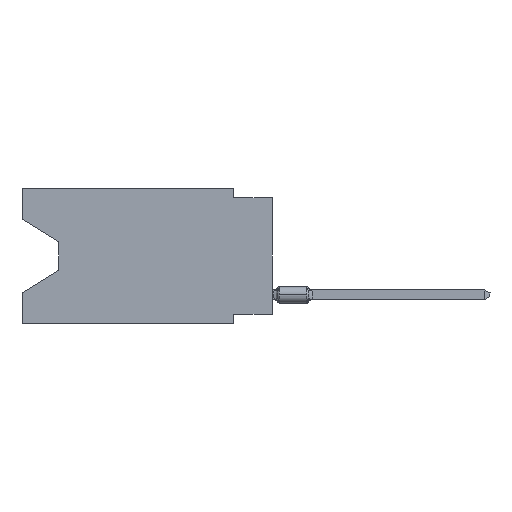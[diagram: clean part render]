
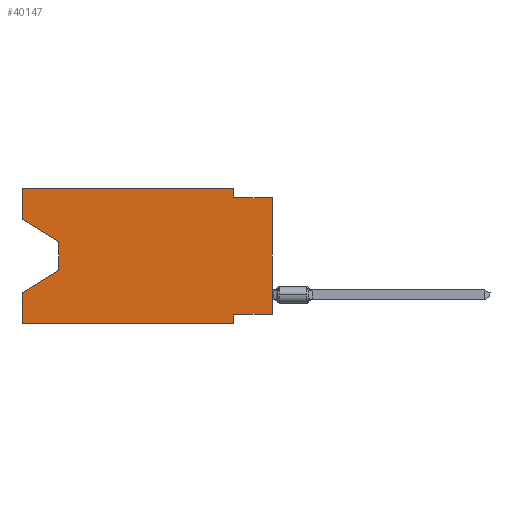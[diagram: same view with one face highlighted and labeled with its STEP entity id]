
A CAD part, left-side view. The second image highlights one B-rep face of the part: STEP entity #40147.
In plain terms, the highlighted planar face has unit normal (-1, 0, 0).
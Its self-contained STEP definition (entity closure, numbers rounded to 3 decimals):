
#376 = DIRECTION ( 'NONE',  ( 0., 0.855, -0.519 ) ) ;
#2074 = EDGE_CURVE ( 'NONE', #8241, #29159, #5861, .T. ) ;
#2849 = CARTESIAN_POINT ( 'NONE',  ( 0., 16.383, -6.852 ) ) ;
#2968 = CARTESIAN_POINT ( 'NONE',  ( 0., 16.383, 0. ) ) ;
#3019 = EDGE_CURVE ( 'NONE', #36247, #46033, #17302, .T. ) ;
#3469 = ORIENTED_EDGE ( 'NONE', *, *, #37032, .T. ) ;
#3727 = CARTESIAN_POINT ( 'NONE',  ( 0., 13.97, -5.385 ) ) ;
#4745 = VERTEX_POINT ( 'NONE', #33444 ) ;
#4913 = CARTESIAN_POINT ( 'NONE',  ( 0., 2.54, -0.635 ) ) ;
#5861 = LINE ( 'NONE', #44570, #18632 ) ;
#6766 = VECTOR ( 'NONE', #48498, 1000. ) ;
#6932 = EDGE_CURVE ( 'NONE', #23714, #14240, #28679, .T. ) ;
#8034 = CARTESIAN_POINT ( 'NONE',  ( 0., 16.383, -8.89 ) ) ;
#8043 = DIRECTION ( 'NONE',  ( 0., 0., -1. ) ) ;
#8229 = VERTEX_POINT ( 'NONE', #39587 ) ;
#8241 = VERTEX_POINT ( 'NONE', #35573 ) ;
#8360 = ORIENTED_EDGE ( 'NONE', *, *, #20843, .T. ) ;
#8700 = AXIS2_PLACEMENT_3D ( 'NONE', #2968, #31608, #11507 ) ;
#9347 = CARTESIAN_POINT ( 'NONE',  ( 0., 16.383, 0. ) ) ;
#9690 = ORIENTED_EDGE ( 'NONE', *, *, #22733, .F. ) ;
#9769 = DIRECTION ( 'NONE',  ( 0., 0., -1. ) ) ;
#10174 = CARTESIAN_POINT ( 'NONE',  ( 0., 0., 0. ) ) ;
#10528 = FACE_OUTER_BOUND ( 'NONE', #45852, .T. ) ;
#10813 = VECTOR ( 'NONE', #36239, 1000. ) ;
#11239 = ORIENTED_EDGE ( 'NONE', *, *, #6932, .F. ) ;
#11507 = DIRECTION ( 'NONE',  ( 0., 0., -1. ) ) ;
#11816 = LINE ( 'NONE', #42480, #31564 ) ;
#14240 = VERTEX_POINT ( 'NONE', #2849 ) ;
#14755 = EDGE_CURVE ( 'NONE', #29159, #14240, #19476, .T. ) ;
#15243 = VECTOR ( 'NONE', #36760, 1000. ) ;
#15750 = ORIENTED_EDGE ( 'NONE', *, *, #35607, .T. ) ;
#16802 = CARTESIAN_POINT ( 'NONE',  ( 0., 2.54, -8.89 ) ) ;
#17302 = LINE ( 'NONE', #44196, #18596 ) ;
#17561 = DIRECTION ( 'NONE',  ( 0., -1., 0. ) ) ;
#18596 = VECTOR ( 'NONE', #17561, 1000. ) ;
#18632 = VECTOR ( 'NONE', #21186, 1000. ) ;
#19333 = ORIENTED_EDGE ( 'NONE', *, *, #14755, .T. ) ;
#19476 = LINE ( 'NONE', #34807, #44686 ) ;
#20001 = CARTESIAN_POINT ( 'NONE',  ( 0., 16.383, 0. ) ) ;
#20843 = EDGE_CURVE ( 'NONE', #23714, #33346, #42471, .T. ) ;
#20923 = ORIENTED_EDGE ( 'NONE', *, *, #45605, .F. ) ;
#21057 = CARTESIAN_POINT ( 'NONE',  ( 0., 2.54, -8.89 ) ) ;
#21186 = DIRECTION ( 'NONE',  ( 0., 0., -1. ) ) ;
#21317 = DIRECTION ( 'NONE',  ( 0., -1., 0. ) ) ;
#22002 = EDGE_CURVE ( 'NONE', #8229, #36247, #11816, .T. ) ;
#22342 = VECTOR ( 'NONE', #21317, 1000. ) ;
#22733 = EDGE_CURVE ( 'NONE', #4745, #39158, #35975, .T. ) ;
#23513 = ORIENTED_EDGE ( 'NONE', *, *, #25412, .F. ) ;
#23714 = VERTEX_POINT ( 'NONE', #39751 ) ;
#25077 = LINE ( 'NONE', #40437, #22342 ) ;
#25412 = EDGE_CURVE ( 'NONE', #41017, #36835, #32747, .T. ) ;
#25479 = DIRECTION ( 'NONE',  ( 0., 0., 1. ) ) ;
#25672 = CARTESIAN_POINT ( 'NONE',  ( 0., 2.54, -8.255 ) ) ;
#25822 = PLANE ( 'NONE',  #8700 ) ;
#27395 = CARTESIAN_POINT ( 'NONE',  ( 0., 16.383, -2.038 ) ) ;
#27652 = LINE ( 'NONE', #27395, #29356 ) ;
#28679 = LINE ( 'NONE', #9347, #10813 ) ;
#29159 = VERTEX_POINT ( 'NONE', #3727 ) ;
#29356 = VECTOR ( 'NONE', #31698, 1000. ) ;
#29930 = VECTOR ( 'NONE', #47234, 1000. ) ;
#30424 = CARTESIAN_POINT ( 'NONE',  ( 0., 0., -8.255 ) ) ;
#31564 = VECTOR ( 'NONE', #8043, 1000. ) ;
#31608 = DIRECTION ( 'NONE',  ( 1., 0., 0. ) ) ;
#31698 = DIRECTION ( 'NONE',  ( 0., -0.855, -0.519 ) ) ;
#32747 = LINE ( 'NONE', #37244, #15243 ) ;
#33183 = CARTESIAN_POINT ( 'NONE',  ( 0., 16.383, 0. ) ) ;
#33346 = VERTEX_POINT ( 'NONE', #16802 ) ;
#33386 = VECTOR ( 'NONE', #25479, 1000. ) ;
#33444 = CARTESIAN_POINT ( 'NONE',  ( 0., 16.383, -2.038 ) ) ;
#34807 = CARTESIAN_POINT ( 'NONE',  ( 0., 13.97, -5.385 ) ) ;
#35027 = ORIENTED_EDGE ( 'NONE', *, *, #2074, .T. ) ;
#35573 = CARTESIAN_POINT ( 'NONE',  ( 0., 13.97, -3.505 ) ) ;
#35607 = EDGE_CURVE ( 'NONE', #41017, #46033, #44588, .T. ) ;
#35637 = ORIENTED_EDGE ( 'NONE', *, *, #45302, .F. ) ;
#35807 = CARTESIAN_POINT ( 'NONE',  ( 0., 0., -0.635 ) ) ;
#35975 = LINE ( 'NONE', #33183, #6766 ) ;
#36239 = DIRECTION ( 'NONE',  ( 0., 0., 1. ) ) ;
#36247 = VERTEX_POINT ( 'NONE', #4913 ) ;
#36760 = DIRECTION ( 'NONE',  ( 0., 1., 0. ) ) ;
#36835 = VERTEX_POINT ( 'NONE', #25672 ) ;
#37032 = EDGE_CURVE ( 'NONE', #4745, #8241, #27652, .T. ) ;
#37244 = CARTESIAN_POINT ( 'NONE',  ( 0., 0., -8.255 ) ) ;
#39158 = VERTEX_POINT ( 'NONE', #20001 ) ;
#39587 = CARTESIAN_POINT ( 'NONE',  ( 0., 2.54, 0. ) ) ;
#39751 = CARTESIAN_POINT ( 'NONE',  ( 0., 16.383, -8.89 ) ) ;
#40147 = ADVANCED_FACE ( 'NONE', ( #10528 ), #25822, .F. ) ;
#40437 = CARTESIAN_POINT ( 'NONE',  ( 0., 16.383, 0. ) ) ;
#41017 = VERTEX_POINT ( 'NONE', #30424 ) ;
#41159 = LINE ( 'NONE', #21057, #45660 ) ;
#42471 = LINE ( 'NONE', #8034, #29930 ) ;
#42480 = CARTESIAN_POINT ( 'NONE',  ( 0., 2.54, 0. ) ) ;
#44196 = CARTESIAN_POINT ( 'NONE',  ( 0., 0., -0.635 ) ) ;
#44409 = ORIENTED_EDGE ( 'NONE', *, *, #22002, .F. ) ;
#44570 = CARTESIAN_POINT ( 'NONE',  ( 0., 13.97, -3.505 ) ) ;
#44588 = LINE ( 'NONE', #10174, #33386 ) ;
#44686 = VECTOR ( 'NONE', #376, 1000. ) ;
#45302 = EDGE_CURVE ( 'NONE', #39158, #8229, #25077, .T. ) ;
#45605 = EDGE_CURVE ( 'NONE', #36835, #33346, #41159, .T. ) ;
#45660 = VECTOR ( 'NONE', #9769, 1000. ) ;
#45852 = EDGE_LOOP ( 'NONE', ( #3469, #35027, #19333, #11239, #8360, #20923, #23513, #15750, #48940, #44409, #35637, #9690 ) ) ;
#46033 = VERTEX_POINT ( 'NONE', #35807 ) ;
#47234 = DIRECTION ( 'NONE',  ( 0., -1., 0. ) ) ;
#48498 = DIRECTION ( 'NONE',  ( 0., 0., 1. ) ) ;
#48940 = ORIENTED_EDGE ( 'NONE', *, *, #3019, .F. ) ;
